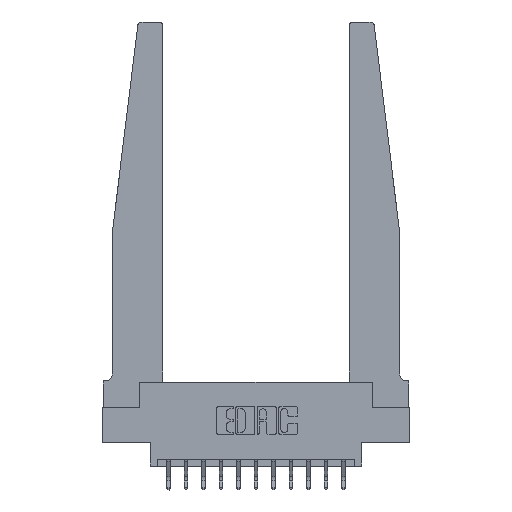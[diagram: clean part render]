
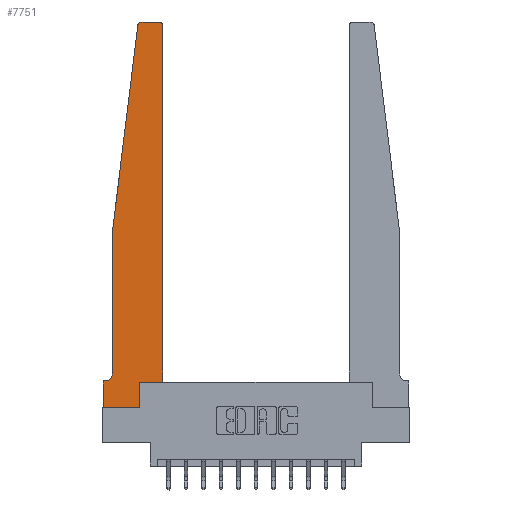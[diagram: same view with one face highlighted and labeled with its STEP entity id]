
A CAD part, top view. The second image highlights one B-rep face of the part: STEP entity #7751.
In plain terms, the highlighted planar face has unit normal (0, 0, 1).
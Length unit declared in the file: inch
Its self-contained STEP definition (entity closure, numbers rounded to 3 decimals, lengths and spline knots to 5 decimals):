
#253 = DIRECTION ( 'NONE',  ( 0., 1., 0. ) ) ;
#317 = VECTOR ( 'NONE', #5490, 39.37008 ) ;
#338 = DIRECTION ( 'NONE',  ( 0., -1., 0. ) ) ;
#380 = CARTESIAN_POINT ( 'NONE',  ( 0.015, 0.2375, 0.37 ) ) ;
#559 = DIRECTION ( 'NONE',  ( 1., 0., 0. ) ) ;
#870 = LINE ( 'NONE', #14006, #11458 ) ;
#1161 = ORIENTED_EDGE ( 'NONE', *, *, #12214, .T. ) ;
#1521 = VERTEX_POINT ( 'NONE', #15059 ) ;
#1708 = DIRECTION ( 'NONE',  ( -1., 0., 0. ) ) ;
#1933 = DIRECTION ( 'NONE',  ( 0., 0., 1. ) ) ;
#2134 = VECTOR ( 'NONE', #253, 39.37008 ) ;
#2296 = PLANE ( 'NONE',  #4363 ) ;
#2433 = VERTEX_POINT ( 'NONE', #11693 ) ;
#2580 = VERTEX_POINT ( 'NONE', #14488 ) ;
#2864 = ORIENTED_EDGE ( 'NONE', *, *, #3504, .T. ) ;
#3088 = CARTESIAN_POINT ( 'NONE',  ( 0.425, 0.18, 0.37 ) ) ;
#3182 = CARTESIAN_POINT ( 'NONE',  ( 0.425, 0.18, 0.37 ) ) ;
#3256 = VERTEX_POINT ( 'NONE', #3808 ) ;
#3342 = VECTOR ( 'NONE', #14999, 39.37008 ) ;
#3504 = EDGE_CURVE ( 'NONE', #2433, #7889, #7827, .T. ) ;
#3641 = CARTESIAN_POINT ( 'NONE',  ( 0.065, 0.1875, 0.37 ) ) ;
#3765 = LINE ( 'NONE', #9240, #317 ) ;
#3808 = CARTESIAN_POINT ( 'NONE',  ( 0., 0.1875, 0.37 ) ) ;
#4059 = VECTOR ( 'NONE', #10682, 39.37008 ) ;
#4089 = ORIENTED_EDGE ( 'NONE', *, *, #7767, .T. ) ;
#4363 = AXIS2_PLACEMENT_3D ( 'NONE', #7379, #4871, #13750 ) ;
#4666 = LINE ( 'NONE', #3182, #8029 ) ;
#4815 = VECTOR ( 'NONE', #15161, 39.37008 ) ;
#4871 = DIRECTION ( 'NONE',  ( 0., 0., 1. ) ) ;
#4909 = CARTESIAN_POINT ( 'NONE',  ( 0.395, 2.75, 0.37 ) ) ;
#5010 = EDGE_CURVE ( 'NONE', #12735, #2580, #7402, .T. ) ;
#5134 = ORIENTED_EDGE ( 'NONE', *, *, #6789, .T. ) ;
#5173 = VERTEX_POINT ( 'NONE', #9191 ) ;
#5244 = CARTESIAN_POINT ( 'NONE',  ( 0.065, 0.2375, 0.37 ) ) ;
#5376 = ORIENTED_EDGE ( 'NONE', *, *, #6251, .T. ) ;
#5490 = DIRECTION ( 'NONE',  ( -0.122, -0.992, 0. ) ) ;
#5572 = CARTESIAN_POINT ( 'NONE',  ( 0., 0., 0.37 ) ) ;
#5580 = DIRECTION ( 'NONE',  ( 0., 0., 1. ) ) ;
#5615 = AXIS2_PLACEMENT_3D ( 'NONE', #13176, #5580, #14422 ) ;
#5617 = EDGE_LOOP ( 'NONE', ( #6514, #6473, #5376, #6778, #5134, #4089, #8209, #1161, #14512, #9835, #2864, #15530 ) ) ;
#6251 = EDGE_CURVE ( 'NONE', #16436, #5173, #3765, .T. ) ;
#6334 = CARTESIAN_POINT ( 'NONE',  ( 0.25, 2.75, 0.37 ) ) ;
#6473 = ORIENTED_EDGE ( 'NONE', *, *, #6898, .T. ) ;
#6514 = ORIENTED_EDGE ( 'NONE', *, *, #5010, .T. ) ;
#6730 = DIRECTION ( 'NONE',  ( 0., -1., 0. ) ) ;
#6764 = CARTESIAN_POINT ( 'NONE',  ( 0.065, 1.25, 0.37 ) ) ;
#6778 = ORIENTED_EDGE ( 'NONE', *, *, #8070, .T. ) ;
#6789 = EDGE_CURVE ( 'NONE', #14459, #10071, #13101, .T. ) ;
#6898 = EDGE_CURVE ( 'NONE', #2580, #16436, #15240, .T. ) ;
#7057 = CARTESIAN_POINT ( 'NONE',  ( 0.015, 0.1875, 0.37 ) ) ;
#7132 = FACE_OUTER_BOUND ( 'NONE', #5617, .T. ) ;
#7379 = CARTESIAN_POINT ( 'NONE',  ( 0., 0.1875, 0.37 ) ) ;
#7402 = LINE ( 'NONE', #6334, #4815 ) ;
#7411 = EDGE_CURVE ( 'NONE', #1521, #7469, #8514, .T. ) ;
#7459 = EDGE_CURVE ( 'NONE', #3256, #9313, #11901, .T. ) ;
#7469 = VERTEX_POINT ( 'NONE', #13100 ) ;
#7751 = ADVANCED_FACE ( 'NONE', ( #7132 ), #2296, .T. ) ;
#7767 = EDGE_CURVE ( 'NONE', #10071, #3256, #10060, .T. ) ;
#7827 = LINE ( 'NONE', #3088, #4059 ) ;
#7889 = VERTEX_POINT ( 'NONE', #8958 ) ;
#7930 = CARTESIAN_POINT ( 'NONE',  ( 0.2605, 0.18, 0.37 ) ) ;
#8029 = VECTOR ( 'NONE', #559, 39.37008 ) ;
#8070 = EDGE_CURVE ( 'NONE', #5173, #14459, #16188, .T. ) ;
#8209 = ORIENTED_EDGE ( 'NONE', *, *, #7459, .T. ) ;
#8514 = LINE ( 'NONE', #7930, #2134 ) ;
#8958 = CARTESIAN_POINT ( 'NONE',  ( 0.425, 2.72, 0.37 ) ) ;
#9191 = CARTESIAN_POINT ( 'NONE',  ( 0.065, 1.25, 0.37 ) ) ;
#9240 = CARTESIAN_POINT ( 'NONE',  ( 0.065, 1.25, 0.37 ) ) ;
#9313 = VERTEX_POINT ( 'NONE', #5572 ) ;
#9326 = DIRECTION ( 'NONE',  ( 0., 0., -1. ) ) ;
#9548 = CARTESIAN_POINT ( 'NONE',  ( 0.27653, 2.72, 0.37 ) ) ;
#9674 = CARTESIAN_POINT ( 'NONE',  ( 0.24675, 2.72367, 0.37 ) ) ;
#9835 = ORIENTED_EDGE ( 'NONE', *, *, #14718, .T. ) ;
#10060 = LINE ( 'NONE', #3641, #3342 ) ;
#10071 = VERTEX_POINT ( 'NONE', #7057 ) ;
#10682 = DIRECTION ( 'NONE',  ( 0., 1., 0. ) ) ;
#10836 = DIRECTION ( 'NONE',  ( 1., 0., 0. ) ) ;
#11458 = VECTOR ( 'NONE', #15267, 39.37008 ) ;
#11693 = CARTESIAN_POINT ( 'NONE',  ( 0.425, 0.18, 0.37 ) ) ;
#11901 = LINE ( 'NONE', #14295, #14443 ) ;
#12214 = EDGE_CURVE ( 'NONE', #9313, #1521, #870, .T. ) ;
#12430 = AXIS2_PLACEMENT_3D ( 'NONE', #380, #9326, #1708 ) ;
#12463 = VECTOR ( 'NONE', #338, 39.37008 ) ;
#12735 = VERTEX_POINT ( 'NONE', #4909 ) ;
#13100 = CARTESIAN_POINT ( 'NONE',  ( 0.2605, 0.18, 0.37 ) ) ;
#13101 = CIRCLE ( 'NONE', #12430, 0.05 ) ;
#13176 = CARTESIAN_POINT ( 'NONE',  ( 0.395, 2.72, 0.37 ) ) ;
#13750 = DIRECTION ( 'NONE',  ( 1., 0., 0. ) ) ;
#14006 = CARTESIAN_POINT ( 'NONE',  ( 0., 0., 0.37 ) ) ;
#14295 = CARTESIAN_POINT ( 'NONE',  ( 0., 0., 0.37 ) ) ;
#14422 = DIRECTION ( 'NONE',  ( 1., 0., 0. ) ) ;
#14443 = VECTOR ( 'NONE', #6730, 39.37008 ) ;
#14459 = VERTEX_POINT ( 'NONE', #5244 ) ;
#14488 = CARTESIAN_POINT ( 'NONE',  ( 0.27653, 2.75, 0.37 ) ) ;
#14512 = ORIENTED_EDGE ( 'NONE', *, *, #7411, .T. ) ;
#14633 = EDGE_CURVE ( 'NONE', #7889, #12735, #15561, .T. ) ;
#14718 = EDGE_CURVE ( 'NONE', #7469, #2433, #4666, .T. ) ;
#14999 = DIRECTION ( 'NONE',  ( -1., 0., 0. ) ) ;
#15059 = CARTESIAN_POINT ( 'NONE',  ( 0.2605, 0., 0.37 ) ) ;
#15161 = DIRECTION ( 'NONE',  ( -1., 0., 0. ) ) ;
#15240 = CIRCLE ( 'NONE', #15810, 0.03 ) ;
#15267 = DIRECTION ( 'NONE',  ( 1., 0., 0. ) ) ;
#15530 = ORIENTED_EDGE ( 'NONE', *, *, #14633, .T. ) ;
#15561 = CIRCLE ( 'NONE', #5615, 0.03 ) ;
#15810 = AXIS2_PLACEMENT_3D ( 'NONE', #9548, #1933, #10836 ) ;
#16188 = LINE ( 'NONE', #6764, #12463 ) ;
#16436 = VERTEX_POINT ( 'NONE', #9674 ) ;
